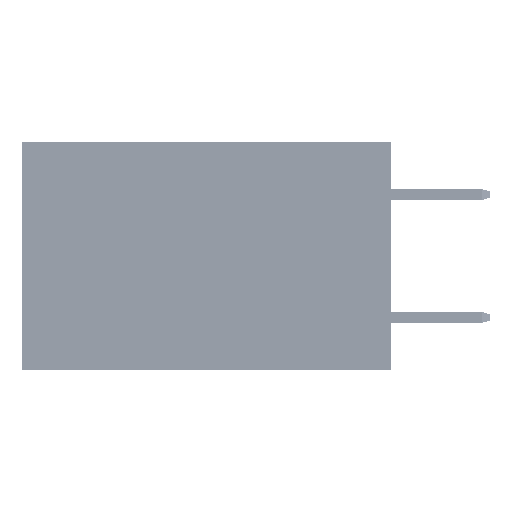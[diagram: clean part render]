
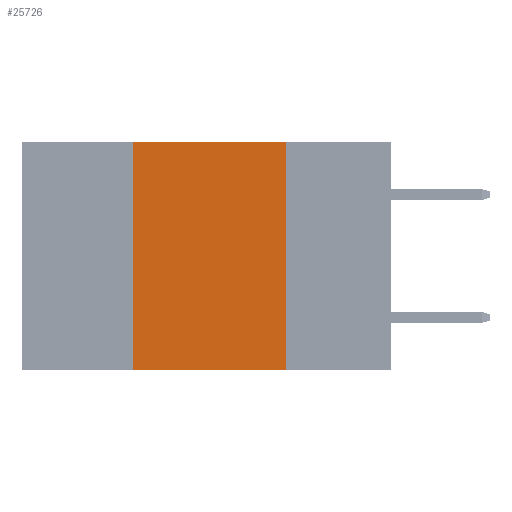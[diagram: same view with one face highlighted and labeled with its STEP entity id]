
A CAD part, left-side view. The second image highlights one B-rep face of the part: STEP entity #25726.
In plain terms, the highlighted planar face has unit normal (-1, 0, 0).
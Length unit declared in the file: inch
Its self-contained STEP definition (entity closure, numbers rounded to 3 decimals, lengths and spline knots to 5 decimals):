
#76 = CARTESIAN_POINT ( 'NONE',  ( 0., 0.6, 0. ) ) ;
#2010 = VECTOR ( 'NONE', #43212, 39.37008 ) ;
#4548 = VECTOR ( 'NONE', #42747, 39.37008 ) ;
#4566 = EDGE_CURVE ( 'NONE', #37872, #29067, #11182, .T. ) ;
#11182 = LINE ( 'NONE', #42494, #4548 ) ;
#11512 = CARTESIAN_POINT ( 'NONE',  ( 0., 0.17, 0. ) ) ;
#11922 = PLANE ( 'NONE',  #30727 ) ;
#11966 = ORIENTED_EDGE ( 'NONE', *, *, #42116, .F. ) ;
#13176 = VERTEX_POINT ( 'NONE', #14352 ) ;
#14352 = CARTESIAN_POINT ( 'NONE',  ( 0., 0.42, -0.37 ) ) ;
#16198 = EDGE_LOOP ( 'NONE', ( #49477, #38141, #11966, #19919 ) ) ;
#16755 = DIRECTION ( 'NONE',  ( 0., 0., 1. ) ) ;
#17007 = LINE ( 'NONE', #28099, #32388 ) ;
#19919 = ORIENTED_EDGE ( 'NONE', *, *, #49702, .T. ) ;
#25726 = ADVANCED_FACE ( 'NONE', ( #31083 ), #11922, .F. ) ;
#26538 = LINE ( 'NONE', #43958, #2010 ) ;
#27048 = DIRECTION ( 'NONE',  ( 1., 0., 0. ) ) ;
#28099 = CARTESIAN_POINT ( 'NONE',  ( 0., 0.42, 0. ) ) ;
#29067 = VERTEX_POINT ( 'NONE', #32849 ) ;
#29471 = CARTESIAN_POINT ( 'NONE',  ( 0., 0.42, 0. ) ) ;
#30727 = AXIS2_PLACEMENT_3D ( 'NONE', #76, #27048, #38433 ) ;
#31083 = FACE_OUTER_BOUND ( 'NONE', #16198, .T. ) ;
#31221 = LINE ( 'NONE', #43852, #49564 ) ;
#32388 = VECTOR ( 'NONE', #16755, 39.37008 ) ;
#32849 = CARTESIAN_POINT ( 'NONE',  ( 0., 0.17, -0.37 ) ) ;
#37872 = VERTEX_POINT ( 'NONE', #11512 ) ;
#38141 = ORIENTED_EDGE ( 'NONE', *, *, #47654, .F. ) ;
#38433 = DIRECTION ( 'NONE',  ( 0., 0., -1. ) ) ;
#42116 = EDGE_CURVE ( 'NONE', #13176, #48124, #17007, .T. ) ;
#42494 = CARTESIAN_POINT ( 'NONE',  ( 0., 0.17, 0. ) ) ;
#42747 = DIRECTION ( 'NONE',  ( 0., 0., -1. ) ) ;
#43212 = DIRECTION ( 'NONE',  ( 0., -1., 0. ) ) ;
#43600 = DIRECTION ( 'NONE',  ( 0., -1., 0. ) ) ;
#43852 = CARTESIAN_POINT ( 'NONE',  ( 0., 0.6, -0.37 ) ) ;
#43958 = CARTESIAN_POINT ( 'NONE',  ( 0., 0.6, 0. ) ) ;
#47654 = EDGE_CURVE ( 'NONE', #48124, #37872, #26538, .T. ) ;
#48124 = VERTEX_POINT ( 'NONE', #29471 ) ;
#49477 = ORIENTED_EDGE ( 'NONE', *, *, #4566, .F. ) ;
#49564 = VECTOR ( 'NONE', #43600, 39.37008 ) ;
#49702 = EDGE_CURVE ( 'NONE', #13176, #29067, #31221, .T. ) ;
